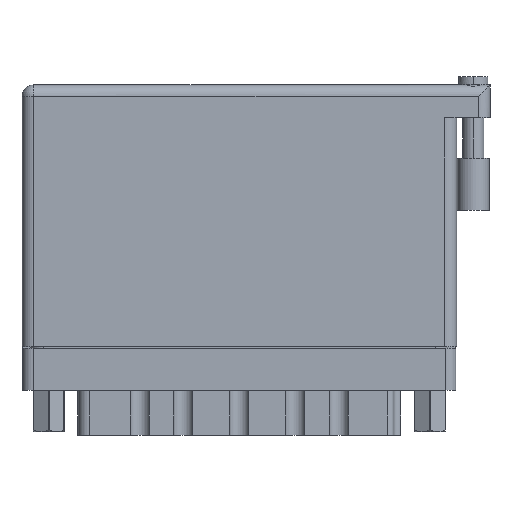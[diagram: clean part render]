
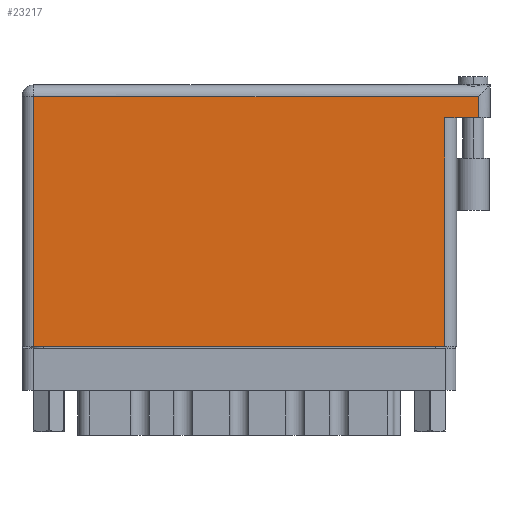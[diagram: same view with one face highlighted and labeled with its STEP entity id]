
A CAD part, front view. The second image highlights one B-rep face of the part: STEP entity #23217.
In plain terms, the highlighted face is planar.
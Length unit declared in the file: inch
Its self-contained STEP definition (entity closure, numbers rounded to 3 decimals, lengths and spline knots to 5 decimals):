
#2035 = CARTESIAN_POINT ( 'NONE',  ( 0.07, 0., 0. ) ) ;
#2759 = ORIENTED_EDGE ( 'NONE', *, *, #8420, .T. ) ;
#4054 = CARTESIAN_POINT ( 'NONE',  ( 2.73, 1.369, 0. ) ) ;
#4968 = DIRECTION ( 'NONE',  ( 0., 0., -1. ) ) ;
#6892 = VECTOR ( 'NONE', #43564, 39.37008 ) ;
#7013 = CARTESIAN_POINT ( 'NONE',  ( 2.73, 1.496, 0. ) ) ;
#8420 = EDGE_CURVE ( 'NONE', #52120, #33399, #57792, .T. ) ;
#9183 = DIRECTION ( 'NONE',  ( -1., 0., 0. ) ) ;
#11276 = EDGE_CURVE ( 'NONE', #41493, #59361, #13885, .T. ) ;
#11617 = EDGE_CURVE ( 'NONE', #26525, #59361, #40774, .T. ) ;
#13036 = DIRECTION ( 'NONE',  ( 0., 1., 0. ) ) ;
#13437 = ORIENTED_EDGE ( 'NONE', *, *, #54842, .T. ) ;
#13831 = VECTOR ( 'NONE', #24856, 39.37008 ) ;
#13885 = LINE ( 'NONE', #15413, #55087 ) ;
#15413 = CARTESIAN_POINT ( 'NONE',  ( 2.53, 1.369, 0. ) ) ;
#18830 = VECTOR ( 'NONE', #33482, 39.37008 ) ;
#19368 = EDGE_CURVE ( 'NONE', #26525, #52120, #40994, .T. ) ;
#19425 = LINE ( 'NONE', #31063, #60620 ) ;
#20418 = DIRECTION ( 'NONE',  ( 0., 1., 0. ) ) ;
#21808 = LINE ( 'NONE', #52599, #18830 ) ;
#22679 = CARTESIAN_POINT ( 'NONE',  ( 2.53, 1.369, 0. ) ) ;
#23217 = ADVANCED_FACE ( 'NONE', ( #30750 ), #57702, .F. ) ;
#24856 = DIRECTION ( 'NONE',  ( -1., 0., 0. ) ) ;
#25089 = EDGE_LOOP ( 'NONE', ( #57522, #46968, #27207, #47972, #2759, #13437 ) ) ;
#26525 = VERTEX_POINT ( 'NONE', #4054 ) ;
#27207 = ORIENTED_EDGE ( 'NONE', *, *, #11617, .F. ) ;
#29714 = VECTOR ( 'NONE', #13036, 39.37008 ) ;
#30750 = FACE_OUTER_BOUND ( 'NONE', #25089, .T. ) ;
#31063 = CARTESIAN_POINT ( 'NONE',  ( 0., 0., 0. ) ) ;
#33399 = VERTEX_POINT ( 'NONE', #50570 ) ;
#33482 = DIRECTION ( 'NONE',  ( 0., -1., 0. ) ) ;
#37087 = VERTEX_POINT ( 'NONE', #2035 ) ;
#39321 = CARTESIAN_POINT ( 'NONE',  ( 2.8, 1.369, 0. ) ) ;
#40774 = LINE ( 'NONE', #39321, #13831 ) ;
#40994 = LINE ( 'NONE', #56546, #29714 ) ;
#41493 = VERTEX_POINT ( 'NONE', #44981 ) ;
#43564 = DIRECTION ( 'NONE',  ( -1., 0., 0. ) ) ;
#44981 = CARTESIAN_POINT ( 'NONE',  ( 2.53, 0., 0. ) ) ;
#45998 = DIRECTION ( 'NONE',  ( 1., 0., 0. ) ) ;
#46968 = ORIENTED_EDGE ( 'NONE', *, *, #11276, .T. ) ;
#47675 = CARTESIAN_POINT ( 'NONE',  ( 0., 1.566, 0. ) ) ;
#47972 = ORIENTED_EDGE ( 'NONE', *, *, #19368, .T. ) ;
#50570 = CARTESIAN_POINT ( 'NONE',  ( 0.07, 1.496, 0. ) ) ;
#52120 = VERTEX_POINT ( 'NONE', #7013 ) ;
#52599 = CARTESIAN_POINT ( 'NONE',  ( 0.07, 0., 0. ) ) ;
#53847 = CARTESIAN_POINT ( 'NONE',  ( 0., 1.496, 0. ) ) ;
#54842 = EDGE_CURVE ( 'NONE', #33399, #37087, #21808, .T. ) ;
#55087 = VECTOR ( 'NONE', #20418, 39.37008 ) ;
#55956 = EDGE_CURVE ( 'NONE', #37087, #41493, #19425, .T. ) ;
#56546 = CARTESIAN_POINT ( 'NONE',  ( 2.73, 1.566, 0. ) ) ;
#57522 = ORIENTED_EDGE ( 'NONE', *, *, #55956, .T. ) ;
#57702 = PLANE ( 'NONE',  #59169 ) ;
#57792 = LINE ( 'NONE', #53847, #6892 ) ;
#59169 = AXIS2_PLACEMENT_3D ( 'NONE', #47675, #4968, #9183 ) ;
#59361 = VERTEX_POINT ( 'NONE', #22679 ) ;
#60620 = VECTOR ( 'NONE', #45998, 39.37008 ) ;
